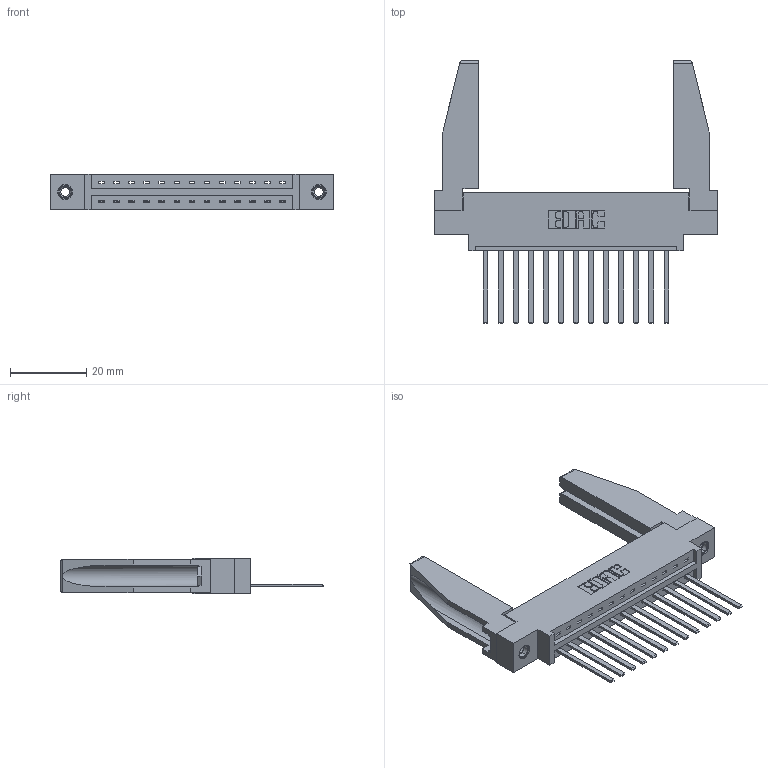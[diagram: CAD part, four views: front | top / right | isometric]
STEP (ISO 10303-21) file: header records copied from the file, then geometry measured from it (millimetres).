
FILE_DESCRIPTION (( 'STEP AP203' ), '1' );
FILE_NAME ('337-013-544-678.STEP', '2019-09-28T02:36:00', ( '' ), ( '' ), 'SwSTEP 2.0', 'SolidWorks 2016', '' );
FILE_SCHEMA (( 'CONFIG_CONTROL_DESIGN' ));
Length unit declared in the file: inch
Products named in the file (5): 345-250-001_345-250-001-102; 337-013-544-678; 337 Part_0.170 Offset - 0.156 Dia-TI; 345-292-001_345-293-144; 307-220-078
Assembly tree (18 placements, depth 2):
  337-013-544-678
    337 Part_0.170 Offset - 0.156 Dia-TI
    345-292-001_345-293-144  x13
    345-250-001_345-250-001-102  x2
    307-220-078  x2
Bounding box: 74.52 x 69.09 x 9.4 mm (x, y, z)
Volume: 11409 mm3; surface area: 11930.6 mm2
Topology: 18 solids, 18 shells, 976 faces, 2863 edges, 1882 vertices
Faces by surface type: plane 704, cylinder 256, cone 12, torus 4
Entity records: 15802 total; most frequent: CARTESIAN_POINT 2743, ORIENTED_EDGE 2648, DIRECTION 2374, EDGE_CURVE 1324, VECTOR 1162, LINE 1162, VERTEX_POINT 876, AXIS2_PLACEMENT_3D 606
